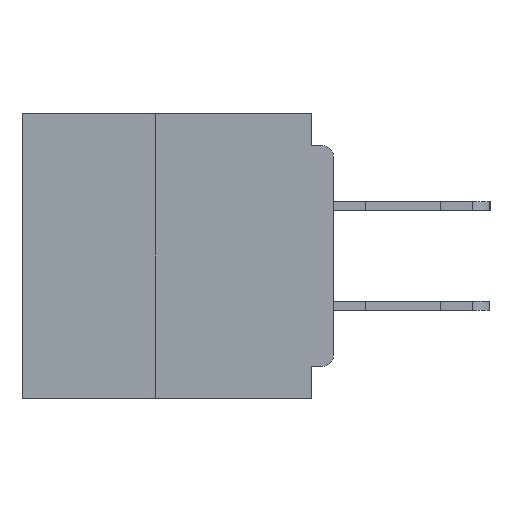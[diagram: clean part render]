
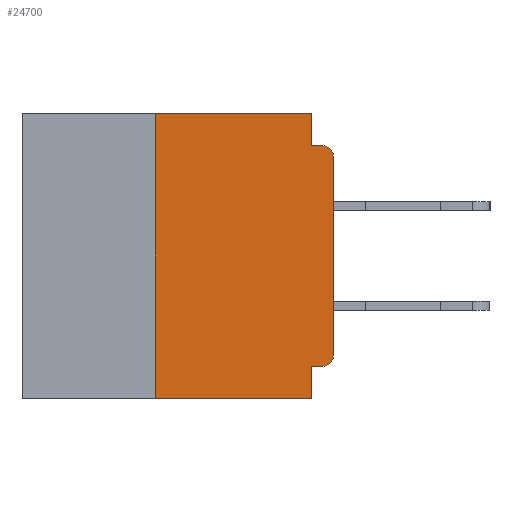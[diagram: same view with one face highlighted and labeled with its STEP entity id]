
A CAD part, left-side view. The second image highlights one B-rep face of the part: STEP entity #24700.
In plain terms, the highlighted planar face has unit normal (-1, 0, 0).
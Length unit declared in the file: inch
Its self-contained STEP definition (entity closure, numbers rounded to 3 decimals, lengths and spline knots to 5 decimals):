
#1047 = VECTOR ( 'NONE', #19377, 39.37008 ) ;
#1715 = EDGE_CURVE ( 'NONE', #15549, #17688, #27777, .T. ) ;
#1974 = DIRECTION ( 'NONE',  ( 0., 1., 0. ) ) ;
#2217 = VERTEX_POINT ( 'NONE', #3678 ) ;
#2704 = CARTESIAN_POINT ( 'NONE',  ( 0., 0.437, 0. ) ) ;
#3282 = CARTESIAN_POINT ( 'NONE',  ( 0., 0.015, -0.045 ) ) ;
#3646 = VECTOR ( 'NONE', #27308, 39.37008 ) ;
#3678 = CARTESIAN_POINT ( 'NONE',  ( 0., 0.031, 0. ) ) ;
#5494 = CARTESIAN_POINT ( 'NONE',  ( 0., 0., -0.06 ) ) ;
#5902 = VECTOR ( 'NONE', #44738, 39.37008 ) ;
#6464 = CARTESIAN_POINT ( 'NONE',  ( 0., 0.015, -0.34 ) ) ;
#8107 = EDGE_LOOP ( 'NONE', ( #17813, #20642, #30949, #22883, #50889, #26994, #20687, #33784, #17144, #21088 ) ) ;
#8270 = VERTEX_POINT ( 'NONE', #27116 ) ;
#8912 = EDGE_CURVE ( 'NONE', #9325, #15549, #35343, .T. ) ;
#9077 = VECTOR ( 'NONE', #1974, 39.37008 ) ;
#9235 = FACE_OUTER_BOUND ( 'NONE', #8107, .T. ) ;
#9325 = VERTEX_POINT ( 'NONE', #32319 ) ;
#9546 = VECTOR ( 'NONE', #33783, 39.37008 ) ;
#9708 = LINE ( 'NONE', #52148, #28994 ) ;
#9748 = LINE ( 'NONE', #24315, #5902 ) ;
#10559 = AXIS2_PLACEMENT_3D ( 'NONE', #6464, #35144, #10578 ) ;
#10578 = DIRECTION ( 'NONE',  ( 0., 0., -1. ) ) ;
#11072 = CARTESIAN_POINT ( 'NONE',  ( 0., 0.031, -0.4 ) ) ;
#12489 = CARTESIAN_POINT ( 'NONE',  ( 0., 0.015, -0.06 ) ) ;
#12668 = EDGE_CURVE ( 'NONE', #31067, #15597, #41818, .T. ) ;
#14521 = LINE ( 'NONE', #2704, #3646 ) ;
#15156 = DIRECTION ( 'NONE',  ( 0., 0., -1. ) ) ;
#15211 = CARTESIAN_POINT ( 'NONE',  ( 0., 0., -0.045 ) ) ;
#15254 = EDGE_CURVE ( 'NONE', #15597, #19245, #43574, .T. ) ;
#15549 = VERTEX_POINT ( 'NONE', #5494 ) ;
#15597 = VERTEX_POINT ( 'NONE', #18057 ) ;
#16613 = DIRECTION ( 'NONE',  ( 0., 0., -1. ) ) ;
#17144 = ORIENTED_EDGE ( 'NONE', *, *, #12668, .F. ) ;
#17555 = CARTESIAN_POINT ( 'NONE',  ( 0., 0.25, -0.4 ) ) ;
#17688 = VERTEX_POINT ( 'NONE', #3282 ) ;
#17813 = ORIENTED_EDGE ( 'NONE', *, *, #8912, .T. ) ;
#18057 = CARTESIAN_POINT ( 'NONE',  ( 0., 0.031, -0.355 ) ) ;
#19245 = VERTEX_POINT ( 'NONE', #50277 ) ;
#19377 = DIRECTION ( 'NONE',  ( 0., -1., 0. ) ) ;
#20642 = ORIENTED_EDGE ( 'NONE', *, *, #1715, .T. ) ;
#20687 = ORIENTED_EDGE ( 'NONE', *, *, #26353, .T. ) ;
#21088 = ORIENTED_EDGE ( 'NONE', *, *, #46746, .T. ) ;
#21715 = CIRCLE ( 'NONE', #10559, 0.015 ) ;
#22883 = ORIENTED_EDGE ( 'NONE', *, *, #42818, .F. ) ;
#24315 = CARTESIAN_POINT ( 'NONE',  ( 0., 0.25, -0.4 ) ) ;
#24700 = ADVANCED_FACE ( 'NONE', ( #9235 ), #40367, .F. ) ;
#26337 = AXIS2_PLACEMENT_3D ( 'NONE', #12489, #41221, #16613 ) ;
#26353 = EDGE_CURVE ( 'NONE', #38115, #19245, #9708, .T. ) ;
#26994 = ORIENTED_EDGE ( 'NONE', *, *, #34536, .F. ) ;
#27116 = CARTESIAN_POINT ( 'NONE',  ( 0., 0.25, 0. ) ) ;
#27308 = DIRECTION ( 'NONE',  ( 0., -1., 0. ) ) ;
#27777 = CIRCLE ( 'NONE', #26337, 0.015 ) ;
#28223 = DIRECTION ( 'NONE',  ( 0., 0., -1. ) ) ;
#28994 = VECTOR ( 'NONE', #43948, 39.37008 ) ;
#29238 = CARTESIAN_POINT ( 'NONE',  ( 0., 0.031, -0.045 ) ) ;
#29540 = EDGE_CURVE ( 'NONE', #8270, #2217, #14521, .T. ) ;
#29710 = CARTESIAN_POINT ( 'NONE',  ( 0., 0., 0. ) ) ;
#30949 = ORIENTED_EDGE ( 'NONE', *, *, #31951, .F. ) ;
#31067 = VERTEX_POINT ( 'NONE', #50412 ) ;
#31951 = EDGE_CURVE ( 'NONE', #32238, #17688, #33774, .T. ) ;
#32238 = VERTEX_POINT ( 'NONE', #29238 ) ;
#32319 = CARTESIAN_POINT ( 'NONE',  ( 0., 0., -0.34 ) ) ;
#33043 = VECTOR ( 'NONE', #48174, 39.37008 ) ;
#33774 = LINE ( 'NONE', #15211, #1047 ) ;
#33783 = DIRECTION ( 'NONE',  ( 0., 0., 1. ) ) ;
#33784 = ORIENTED_EDGE ( 'NONE', *, *, #15254, .F. ) ;
#34536 = EDGE_CURVE ( 'NONE', #38115, #8270, #9748, .T. ) ;
#35144 = DIRECTION ( 'NONE',  ( -1., 0., 0. ) ) ;
#35343 = LINE ( 'NONE', #29710, #9546 ) ;
#36222 = CARTESIAN_POINT ( 'NONE',  ( 0., 0.437, 0. ) ) ;
#38115 = VERTEX_POINT ( 'NONE', #17555 ) ;
#40367 = PLANE ( 'NONE',  #45247 ) ;
#41221 = DIRECTION ( 'NONE',  ( -1., 0., 0. ) ) ;
#41818 = LINE ( 'NONE', #51073, #9077 ) ;
#42256 = VECTOR ( 'NONE', #15156, 39.37008 ) ;
#42818 = EDGE_CURVE ( 'NONE', #2217, #32238, #43982, .T. ) ;
#43574 = LINE ( 'NONE', #11072, #42256 ) ;
#43948 = DIRECTION ( 'NONE',  ( 0., -1., 0. ) ) ;
#43982 = LINE ( 'NONE', #52068, #33043 ) ;
#44738 = DIRECTION ( 'NONE',  ( 0., 0., 1. ) ) ;
#45247 = AXIS2_PLACEMENT_3D ( 'NONE', #36222, #52702, #28223 ) ;
#46746 = EDGE_CURVE ( 'NONE', #31067, #9325, #21715, .T. ) ;
#48174 = DIRECTION ( 'NONE',  ( 0., 0., -1. ) ) ;
#50277 = CARTESIAN_POINT ( 'NONE',  ( 0., 0.031, -0.4 ) ) ;
#50412 = CARTESIAN_POINT ( 'NONE',  ( 0., 0.015, -0.355 ) ) ;
#50889 = ORIENTED_EDGE ( 'NONE', *, *, #29540, .F. ) ;
#51073 = CARTESIAN_POINT ( 'NONE',  ( 0., 0., -0.355 ) ) ;
#52068 = CARTESIAN_POINT ( 'NONE',  ( 0., 0.031, 0. ) ) ;
#52148 = CARTESIAN_POINT ( 'NONE',  ( 0., 0.437, -0.4 ) ) ;
#52702 = DIRECTION ( 'NONE',  ( 1., 0., 0. ) ) ;
